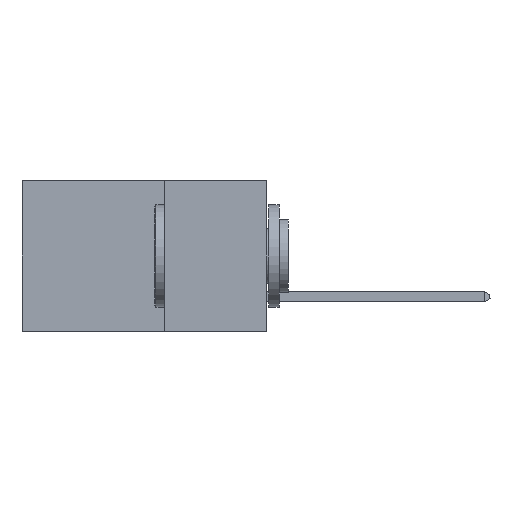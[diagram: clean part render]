
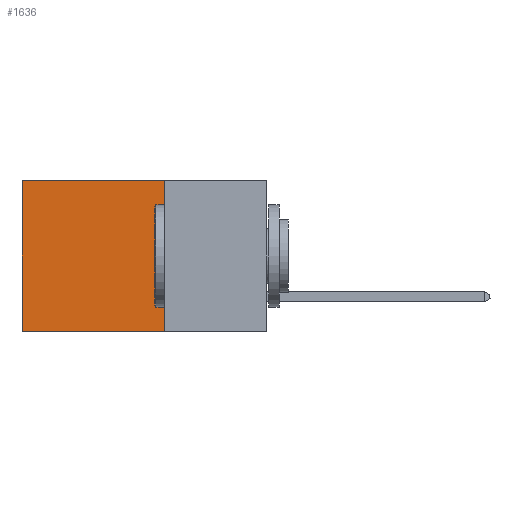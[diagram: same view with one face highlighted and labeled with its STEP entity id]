
A CAD part, left-side view. The second image highlights one B-rep face of the part: STEP entity #1636.
In plain terms, the highlighted planar face has unit normal (-1, 0, 0).
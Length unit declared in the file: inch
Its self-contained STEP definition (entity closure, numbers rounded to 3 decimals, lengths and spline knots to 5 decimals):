
#287 = DIRECTION ( 'NONE',  ( 0., 1., 0. ) ) ;
#940 = LINE ( 'NONE', #1602, #7124 ) ;
#1449 = AXIS2_PLACEMENT_3D ( 'NONE', #9870, #13194, #3516 ) ;
#1581 = CARTESIAN_POINT ( 'NONE',  ( 0.2875, 0.25, 0. ) ) ;
#1602 = CARTESIAN_POINT ( 'NONE',  ( 0.2875, 0.25, -0.37 ) ) ;
#1636 = ADVANCED_FACE ( 'NONE', ( #6257 ), #14688, .F. ) ;
#2069 = EDGE_CURVE ( 'NONE', #8475, #14572, #3347, .T. ) ;
#2376 = CARTESIAN_POINT ( 'NONE',  ( 0.2875, 0.6, 0. ) ) ;
#2650 = VERTEX_POINT ( 'NONE', #9849 ) ;
#3347 = LINE ( 'NONE', #1581, #15601 ) ;
#3516 = DIRECTION ( 'NONE',  ( 0., 0., -1. ) ) ;
#5243 = VECTOR ( 'NONE', #5552, 39.37008 ) ;
#5345 = EDGE_LOOP ( 'NONE', ( #9358, #9570, #9635, #9864 ) ) ;
#5552 = DIRECTION ( 'NONE',  ( 0., 0., -1. ) ) ;
#5615 = DIRECTION ( 'NONE',  ( 0., 0., -1. ) ) ;
#6257 = FACE_OUTER_BOUND ( 'NONE', #5345, .T. ) ;
#7124 = VECTOR ( 'NONE', #287, 39.37008 ) ;
#7489 = DIRECTION ( 'NONE',  ( 0., 1., 0. ) ) ;
#8475 = VERTEX_POINT ( 'NONE', #14517 ) ;
#8850 = LINE ( 'NONE', #11558, #5243 ) ;
#9358 = ORIENTED_EDGE ( 'NONE', *, *, #9867, .T. ) ;
#9570 = ORIENTED_EDGE ( 'NONE', *, *, #10584, .F. ) ;
#9635 = ORIENTED_EDGE ( 'NONE', *, *, #2069, .F. ) ;
#9849 = CARTESIAN_POINT ( 'NONE',  ( 0.2875, 0.6, -0.37 ) ) ;
#9864 = ORIENTED_EDGE ( 'NONE', *, *, #13638, .T. ) ;
#9867 = EDGE_CURVE ( 'NONE', #13540, #2650, #8850, .T. ) ;
#9870 = CARTESIAN_POINT ( 'NONE',  ( 0.2875, 0.25, 0. ) ) ;
#10584 = EDGE_CURVE ( 'NONE', #14572, #2650, #940, .T. ) ;
#11043 = CARTESIAN_POINT ( 'NONE',  ( 0.2875, 0.25, 0. ) ) ;
#11558 = CARTESIAN_POINT ( 'NONE',  ( 0.2875, 0.6, 0. ) ) ;
#12189 = VECTOR ( 'NONE', #7489, 39.37008 ) ;
#13194 = DIRECTION ( 'NONE',  ( 1., 0., 0. ) ) ;
#13540 = VERTEX_POINT ( 'NONE', #2376 ) ;
#13638 = EDGE_CURVE ( 'NONE', #8475, #13540, #15243, .T. ) ;
#14517 = CARTESIAN_POINT ( 'NONE',  ( 0.2875, 0.25, 0. ) ) ;
#14572 = VERTEX_POINT ( 'NONE', #15092 ) ;
#14688 = PLANE ( 'NONE',  #1449 ) ;
#15092 = CARTESIAN_POINT ( 'NONE',  ( 0.2875, 0.25, -0.37 ) ) ;
#15243 = LINE ( 'NONE', #11043, #12189 ) ;
#15601 = VECTOR ( 'NONE', #5615, 39.37008 ) ;
